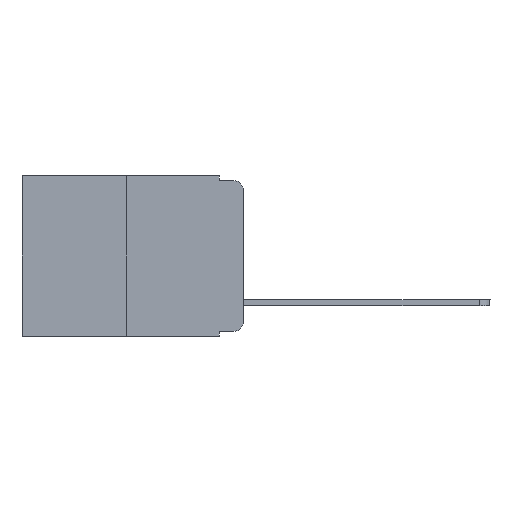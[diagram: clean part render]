
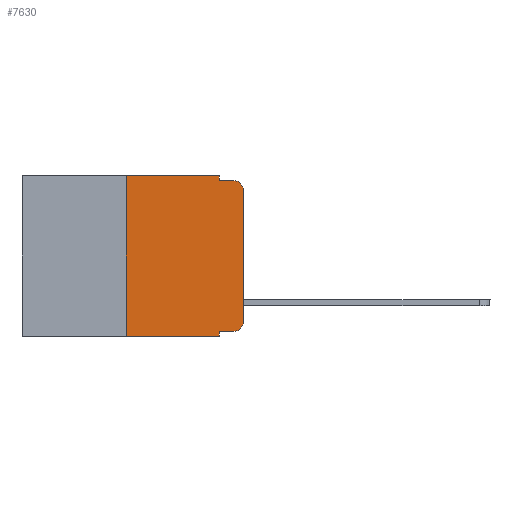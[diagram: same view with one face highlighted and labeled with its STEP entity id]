
A CAD part, left-side view. The second image highlights one B-rep face of the part: STEP entity #7630.
In plain terms, the highlighted planar face has unit normal (-1, 0, 0).
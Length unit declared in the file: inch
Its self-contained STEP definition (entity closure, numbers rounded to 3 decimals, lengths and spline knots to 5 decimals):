
#16 = ORIENTED_EDGE ( 'NONE', *, *, #7536, .F. ) ;
#53 = AXIS2_PLACEMENT_3D ( 'NONE', #3188, #7832, #11396 ) ;
#350 = CARTESIAN_POINT ( 'NONE',  ( 0., 0.02, -0.333 ) ) ;
#667 = CARTESIAN_POINT ( 'NONE',  ( 0., 0., -0.03 ) ) ;
#743 = DIRECTION ( 'NONE',  ( 0., -1., 0. ) ) ;
#774 = LINE ( 'NONE', #9442, #4109 ) ;
#893 = DIRECTION ( 'NONE',  ( 0., -1., 0. ) ) ;
#929 = CIRCLE ( 'NONE', #5203, 0.02 ) ;
#948 = VECTOR ( 'NONE', #893, 39.37008 ) ;
#1011 = LINE ( 'NONE', #6404, #2965 ) ;
#1097 = VECTOR ( 'NONE', #9708, 39.37008 ) ;
#1122 = VERTEX_POINT ( 'NONE', #6274 ) ;
#1317 = VECTOR ( 'NONE', #8616, 39.37008 ) ;
#1528 = LINE ( 'NONE', #5072, #1317 ) ;
#1586 = CARTESIAN_POINT ( 'NONE',  ( 0., 0.02, -0.03 ) ) ;
#2102 = VECTOR ( 'NONE', #743, 39.37008 ) ;
#2257 = EDGE_CURVE ( 'NONE', #5951, #9180, #7072, .T. ) ;
#2442 = VERTEX_POINT ( 'NONE', #11082 ) ;
#2568 = EDGE_CURVE ( 'NONE', #9180, #8103, #774, .T. ) ;
#2658 = CARTESIAN_POINT ( 'NONE',  ( 0., 0.051, 0. ) ) ;
#2965 = VECTOR ( 'NONE', #5486, 39.37008 ) ;
#3188 = CARTESIAN_POINT ( 'NONE',  ( 0., 0.473, 0. ) ) ;
#3335 = ORIENTED_EDGE ( 'NONE', *, *, #4934, .F. ) ;
#3340 = DIRECTION ( 'NONE',  ( 0., 0., -1. ) ) ;
#3348 = CARTESIAN_POINT ( 'NONE',  ( 0., 0., -0.313 ) ) ;
#3366 = CARTESIAN_POINT ( 'NONE',  ( 0., 0.051, 0. ) ) ;
#3476 = LINE ( 'NONE', #2658, #1097 ) ;
#3757 = CARTESIAN_POINT ( 'NONE',  ( 0., 0.473, 0. ) ) ;
#4006 = EDGE_CURVE ( 'NONE', #7306, #4921, #1011, .T. ) ;
#4109 = VECTOR ( 'NONE', #6757, 39.37008 ) ;
#4222 = CARTESIAN_POINT ( 'NONE',  ( 0., 0.051, 0. ) ) ;
#4247 = ORIENTED_EDGE ( 'NONE', *, *, #4006, .F. ) ;
#4295 = FACE_OUTER_BOUND ( 'NONE', #7164, .T. ) ;
#4411 = CARTESIAN_POINT ( 'NONE',  ( 0., 0.051, -0.01 ) ) ;
#4433 = ORIENTED_EDGE ( 'NONE', *, *, #2568, .T. ) ;
#4921 = VERTEX_POINT ( 'NONE', #8828 ) ;
#4934 = EDGE_CURVE ( 'NONE', #11322, #8558, #3476, .T. ) ;
#5072 = CARTESIAN_POINT ( 'NONE',  ( 0., 0.051, -0.333 ) ) ;
#5203 = AXIS2_PLACEMENT_3D ( 'NONE', #1586, #9609, #7738 ) ;
#5486 = DIRECTION ( 'NONE',  ( 0., 0., 1. ) ) ;
#5541 = CARTESIAN_POINT ( 'NONE',  ( 0., 0.473, -0.343 ) ) ;
#5700 = EDGE_CURVE ( 'NONE', #1122, #5951, #1528, .T. ) ;
#5857 = CARTESIAN_POINT ( 'NONE',  ( 0., 0.051, -0.01 ) ) ;
#5951 = VERTEX_POINT ( 'NONE', #350 ) ;
#5963 = AXIS2_PLACEMENT_3D ( 'NONE', #7758, #11313, #3340 ) ;
#6030 = PLANE ( 'NONE',  #53 ) ;
#6274 = CARTESIAN_POINT ( 'NONE',  ( 0., 0.051, -0.333 ) ) ;
#6289 = CARTESIAN_POINT ( 'NONE',  ( 0., 0.051, -0.343 ) ) ;
#6362 = LINE ( 'NONE', #3757, #948 ) ;
#6404 = CARTESIAN_POINT ( 'NONE',  ( 0., 0.25, 0. ) ) ;
#6464 = EDGE_CURVE ( 'NONE', #4921, #11322, #6362, .T. ) ;
#6557 = VERTEX_POINT ( 'NONE', #6289 ) ;
#6757 = DIRECTION ( 'NONE',  ( 0., 0., 1. ) ) ;
#6787 = DIRECTION ( 'NONE',  ( 0., 0., -1. ) ) ;
#7072 = CIRCLE ( 'NONE', #5963, 0.02 ) ;
#7115 = ORIENTED_EDGE ( 'NONE', *, *, #10114, .F. ) ;
#7164 = EDGE_LOOP ( 'NONE', ( #4433, #9260, #16, #3335, #10176, #4247, #8974, #7115, #8362, #10568 ) ) ;
#7306 = VERTEX_POINT ( 'NONE', #10649 ) ;
#7536 = EDGE_CURVE ( 'NONE', #8558, #2442, #11164, .T. ) ;
#7630 = ADVANCED_FACE ( 'NONE', ( #4295 ), #6030, .F. ) ;
#7738 = DIRECTION ( 'NONE',  ( 0., 0., -1. ) ) ;
#7758 = CARTESIAN_POINT ( 'NONE',  ( 0., 0.02, -0.313 ) ) ;
#7832 = DIRECTION ( 'NONE',  ( 1., 0., 0. ) ) ;
#8103 = VERTEX_POINT ( 'NONE', #667 ) ;
#8248 = EDGE_CURVE ( 'NONE', #7306, #6557, #8910, .T. ) ;
#8362 = ORIENTED_EDGE ( 'NONE', *, *, #5700, .T. ) ;
#8558 = VERTEX_POINT ( 'NONE', #4411 ) ;
#8602 = LINE ( 'NONE', #3366, #10598 ) ;
#8616 = DIRECTION ( 'NONE',  ( 0., -1., 0. ) ) ;
#8828 = CARTESIAN_POINT ( 'NONE',  ( 0., 0.25, 0. ) ) ;
#8910 = LINE ( 'NONE', #5541, #10088 ) ;
#8974 = ORIENTED_EDGE ( 'NONE', *, *, #8248, .T. ) ;
#9180 = VERTEX_POINT ( 'NONE', #3348 ) ;
#9260 = ORIENTED_EDGE ( 'NONE', *, *, #9704, .T. ) ;
#9442 = CARTESIAN_POINT ( 'NONE',  ( 0., 0., 0. ) ) ;
#9609 = DIRECTION ( 'NONE',  ( -1., 0., 0. ) ) ;
#9704 = EDGE_CURVE ( 'NONE', #8103, #2442, #929, .T. ) ;
#9708 = DIRECTION ( 'NONE',  ( 0., 0., -1. ) ) ;
#9970 = DIRECTION ( 'NONE',  ( 0., -1., 0. ) ) ;
#10088 = VECTOR ( 'NONE', #9970, 39.37008 ) ;
#10114 = EDGE_CURVE ( 'NONE', #1122, #6557, #8602, .T. ) ;
#10176 = ORIENTED_EDGE ( 'NONE', *, *, #6464, .F. ) ;
#10568 = ORIENTED_EDGE ( 'NONE', *, *, #2257, .T. ) ;
#10598 = VECTOR ( 'NONE', #6787, 39.37008 ) ;
#10649 = CARTESIAN_POINT ( 'NONE',  ( 0., 0.25, -0.343 ) ) ;
#11082 = CARTESIAN_POINT ( 'NONE',  ( 0., 0.02, -0.01 ) ) ;
#11164 = LINE ( 'NONE', #5857, #2102 ) ;
#11313 = DIRECTION ( 'NONE',  ( -1., 0., 0. ) ) ;
#11322 = VERTEX_POINT ( 'NONE', #4222 ) ;
#11396 = DIRECTION ( 'NONE',  ( 0., 0., -1. ) ) ;
